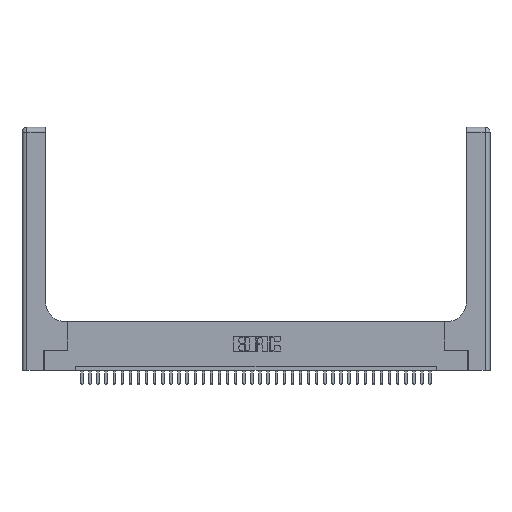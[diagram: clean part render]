
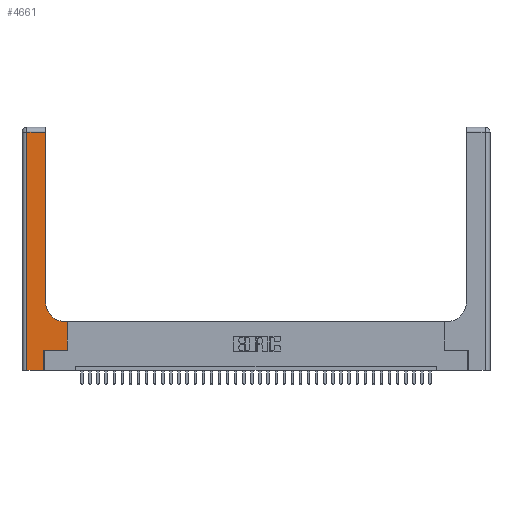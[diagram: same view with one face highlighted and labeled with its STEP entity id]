
A CAD part, top view. The second image highlights one B-rep face of the part: STEP entity #4661.
In plain terms, the highlighted planar face has unit normal (0, 0, 1).
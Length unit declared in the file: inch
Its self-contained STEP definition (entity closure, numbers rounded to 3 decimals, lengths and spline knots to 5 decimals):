
#635 = DIRECTION ( 'NONE',  ( 0., 0., -1. ) ) ;
#640 = DIRECTION ( 'NONE',  ( 1., 0., 0. ) ) ;
#1121 = LINE ( 'NONE', #18300, #19097 ) ;
#1748 = VERTEX_POINT ( 'NONE', #21838 ) ;
#2244 = EDGE_CURVE ( 'NONE', #5664, #6766, #20882, .T. ) ;
#2966 = ORIENTED_EDGE ( 'NONE', *, *, #23670, .T. ) ;
#3633 = PLANE ( 'NONE',  #24533 ) ;
#4661 = ADVANCED_FACE ( 'NONE', ( #36523 ), #3633, .F. ) ;
#4680 = EDGE_CURVE ( 'NONE', #6766, #30045, #32860, .T. ) ;
#5138 = CARTESIAN_POINT ( 'NONE',  ( 0.5415, 0.85, 0.37 ) ) ;
#5664 = VERTEX_POINT ( 'NONE', #15091 ) ;
#6479 = LINE ( 'NONE', #27359, #31356 ) ;
#6701 = DIRECTION ( 'NONE',  ( 0., -1., 0. ) ) ;
#6725 = DIRECTION ( 'NONE',  ( -1., 0., 0. ) ) ;
#6766 = VERTEX_POINT ( 'NONE', #35265 ) ;
#7103 = CIRCLE ( 'NONE', #35792, 0.25 ) ;
#7355 = VERTEX_POINT ( 'NONE', #33617 ) ;
#7855 = VECTOR ( 'NONE', #32983, 39.37008 ) ;
#8367 = ORIENTED_EDGE ( 'NONE', *, *, #12814, .T. ) ;
#8818 = CARTESIAN_POINT ( 'NONE',  ( 0., 2.94, 0.37 ) ) ;
#9937 = CARTESIAN_POINT ( 'NONE',  ( 0., 3., 0.37 ) ) ;
#10348 = VERTEX_POINT ( 'NONE', #34583 ) ;
#10884 = EDGE_CURVE ( 'NONE', #10348, #7355, #27963, .T. ) ;
#11104 = LINE ( 'NONE', #27080, #7855 ) ;
#12176 = LINE ( 'NONE', #8818, #20969 ) ;
#12814 = EDGE_CURVE ( 'NONE', #30328, #10348, #1121, .T. ) ;
#13244 = CARTESIAN_POINT ( 'NONE',  ( 0.5585, 0.25, 0.37 ) ) ;
#14048 = ORIENTED_EDGE ( 'NONE', *, *, #4680, .T. ) ;
#14939 = DIRECTION ( 'NONE',  ( -1., 0., 0. ) ) ;
#15091 = CARTESIAN_POINT ( 'NONE',  ( 0.5585, 0.25, 0.37 ) ) ;
#16715 = VECTOR ( 'NONE', #34757, 39.37008 ) ;
#17295 = VECTOR ( 'NONE', #6725, 39.37008 ) ;
#17775 = ORIENTED_EDGE ( 'NONE', *, *, #22637, .T. ) ;
#18300 = CARTESIAN_POINT ( 'NONE',  ( 0.06, 3., 0.37 ) ) ;
#18388 = EDGE_CURVE ( 'NONE', #1748, #20110, #29520, .T. ) ;
#18650 = DIRECTION ( 'NONE',  ( 0., 1., 0. ) ) ;
#18759 = VECTOR ( 'NONE', #25114, 39.37008 ) ;
#19097 = VECTOR ( 'NONE', #6701, 39.37008 ) ;
#19695 = DIRECTION ( 'NONE',  ( 1., 0., 0. ) ) ;
#19985 = ORIENTED_EDGE ( 'NONE', *, *, #10884, .T. ) ;
#20110 = VERTEX_POINT ( 'NONE', #30950 ) ;
#20882 = LINE ( 'NONE', #13244, #31040 ) ;
#20969 = VECTOR ( 'NONE', #14939, 39.37008 ) ;
#21838 = CARTESIAN_POINT ( 'NONE',  ( 0.2915, 0.85, 0.37 ) ) ;
#21840 = CARTESIAN_POINT ( 'NONE',  ( 0.5415, 0.6, 0.37 ) ) ;
#22206 = EDGE_LOOP ( 'NONE', ( #30188, #17775, #8367, #19985, #2966, #24312, #31262, #14048, #30987 ) ) ;
#22637 = EDGE_CURVE ( 'NONE', #20110, #30328, #12176, .T. ) ;
#23008 = CARTESIAN_POINT ( 'NONE',  ( 0.06, 2.94, 0.37 ) ) ;
#23670 = EDGE_CURVE ( 'NONE', #7355, #25236, #11104, .T. ) ;
#23730 = EDGE_CURVE ( 'NONE', #25236, #5664, #6479, .T. ) ;
#24312 = ORIENTED_EDGE ( 'NONE', *, *, #23730, .T. ) ;
#24395 = CARTESIAN_POINT ( 'NONE',  ( 0.2915, 0.6, 0.37 ) ) ;
#24533 = AXIS2_PLACEMENT_3D ( 'NONE', #9937, #635, #30576 ) ;
#25114 = DIRECTION ( 'NONE',  ( 1., 0., 0. ) ) ;
#25236 = VERTEX_POINT ( 'NONE', #37007 ) ;
#27080 = CARTESIAN_POINT ( 'NONE',  ( 0.269, 0., 0.37 ) ) ;
#27359 = CARTESIAN_POINT ( 'NONE',  ( 0.269, 0.25, 0.37 ) ) ;
#27963 = LINE ( 'NONE', #36119, #18759 ) ;
#28996 = CARTESIAN_POINT ( 'NONE',  ( 0.2915, 3., 0.37 ) ) ;
#29520 = LINE ( 'NONE', #28996, #16715 ) ;
#30045 = VERTEX_POINT ( 'NONE', #21840 ) ;
#30188 = ORIENTED_EDGE ( 'NONE', *, *, #18388, .T. ) ;
#30328 = VERTEX_POINT ( 'NONE', #23008 ) ;
#30576 = DIRECTION ( 'NONE',  ( -1., 0., 0. ) ) ;
#30950 = CARTESIAN_POINT ( 'NONE',  ( 0.2915, 2.94, 0.37 ) ) ;
#30987 = ORIENTED_EDGE ( 'NONE', *, *, #36006, .T. ) ;
#31040 = VECTOR ( 'NONE', #18650, 39.37008 ) ;
#31262 = ORIENTED_EDGE ( 'NONE', *, *, #2244, .T. ) ;
#31356 = VECTOR ( 'NONE', #640, 39.37008 ) ;
#32860 = LINE ( 'NONE', #24395, #17295 ) ;
#32983 = DIRECTION ( 'NONE',  ( 0., 1., 0. ) ) ;
#33617 = CARTESIAN_POINT ( 'NONE',  ( 0.269, 0., 0.37 ) ) ;
#34328 = DIRECTION ( 'NONE',  ( 0., 0., -1. ) ) ;
#34583 = CARTESIAN_POINT ( 'NONE',  ( 0.06, 0., 0.37 ) ) ;
#34757 = DIRECTION ( 'NONE',  ( 0., 1., 0. ) ) ;
#35265 = CARTESIAN_POINT ( 'NONE',  ( 0.5585, 0.6, 0.37 ) ) ;
#35792 = AXIS2_PLACEMENT_3D ( 'NONE', #5138, #34328, #19695 ) ;
#36006 = EDGE_CURVE ( 'NONE', #30045, #1748, #7103, .T. ) ;
#36119 = CARTESIAN_POINT ( 'NONE',  ( 0., 0., 0.37 ) ) ;
#36523 = FACE_OUTER_BOUND ( 'NONE', #22206, .T. ) ;
#37007 = CARTESIAN_POINT ( 'NONE',  ( 0.269, 0.25, 0.37 ) ) ;
